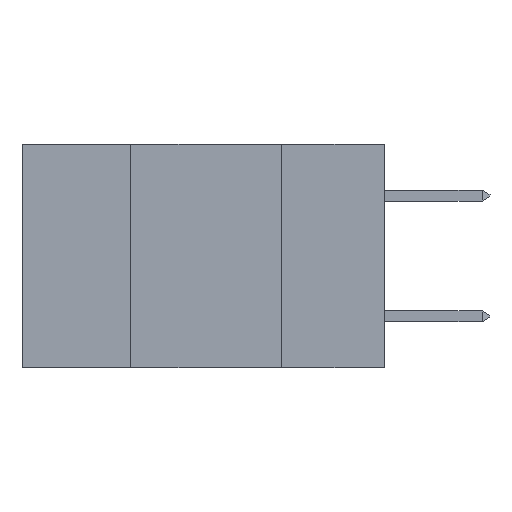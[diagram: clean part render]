
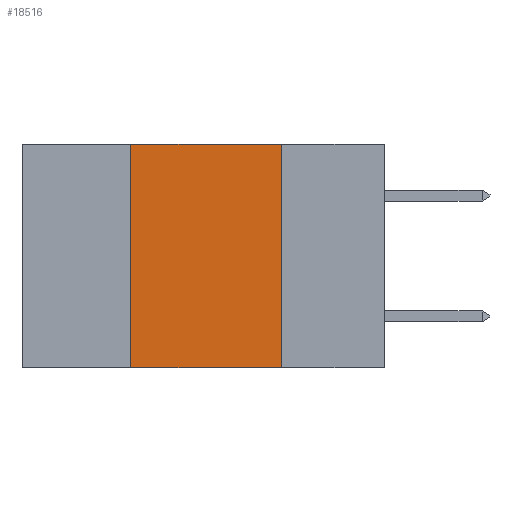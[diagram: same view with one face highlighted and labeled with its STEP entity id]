
A CAD part, left-side view. The second image highlights one B-rep face of the part: STEP entity #18516.
In plain terms, the highlighted planar face has unit normal (-1, 0, 0).
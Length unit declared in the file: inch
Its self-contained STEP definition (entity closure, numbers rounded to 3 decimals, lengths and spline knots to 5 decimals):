
#1096 = LINE ( 'NONE', #18231, #2732 ) ;
#1862 = DIRECTION ( 'NONE',  ( 0., 0., 1. ) ) ;
#2732 = VECTOR ( 'NONE', #21610, 39.37008 ) ;
#2871 = ORIENTED_EDGE ( 'NONE', *, *, #7036, .F. ) ;
#2920 = LINE ( 'NONE', #2976, #15024 ) ;
#2976 = CARTESIAN_POINT ( 'NONE',  ( 0., 0.17, 0. ) ) ;
#3506 = EDGE_CURVE ( 'NONE', #19557, #21065, #7070, .T. ) ;
#3613 = VECTOR ( 'NONE', #1862, 39.37008 ) ;
#3697 = FACE_OUTER_BOUND ( 'NONE', #12694, .T. ) ;
#4032 = DIRECTION ( 'NONE',  ( 0., -1., 0. ) ) ;
#5654 = CARTESIAN_POINT ( 'NONE',  ( 0., 0.6, 0. ) ) ;
#6353 = CARTESIAN_POINT ( 'NONE',  ( 0., 0.6, 0. ) ) ;
#7036 = EDGE_CURVE ( 'NONE', #21065, #18867, #2920, .T. ) ;
#7070 = LINE ( 'NONE', #5654, #15033 ) ;
#7922 = DIRECTION ( 'NONE',  ( 1., 0., 0. ) ) ;
#8069 = DIRECTION ( 'NONE',  ( 0., 0., -1. ) ) ;
#8306 = LINE ( 'NONE', #14078, #3613 ) ;
#8861 = AXIS2_PLACEMENT_3D ( 'NONE', #6353, #7922, #8069 ) ;
#9609 = PLANE ( 'NONE',  #8861 ) ;
#10303 = CARTESIAN_POINT ( 'NONE',  ( 0., 0.17, -0.37 ) ) ;
#10659 = ORIENTED_EDGE ( 'NONE', *, *, #20138, .F. ) ;
#11064 = CARTESIAN_POINT ( 'NONE',  ( 0., 0.17, 0. ) ) ;
#12694 = EDGE_LOOP ( 'NONE', ( #2871, #20544, #10659, #18082 ) ) ;
#14078 = CARTESIAN_POINT ( 'NONE',  ( 0., 0.42, 0. ) ) ;
#15024 = VECTOR ( 'NONE', #15264, 39.37008 ) ;
#15033 = VECTOR ( 'NONE', #4032, 39.37008 ) ;
#15264 = DIRECTION ( 'NONE',  ( 0., 0., -1. ) ) ;
#17601 = VERTEX_POINT ( 'NONE', #18396 ) ;
#18082 = ORIENTED_EDGE ( 'NONE', *, *, #22385, .T. ) ;
#18231 = CARTESIAN_POINT ( 'NONE',  ( 0., 0.6, -0.37 ) ) ;
#18396 = CARTESIAN_POINT ( 'NONE',  ( 0., 0.42, -0.37 ) ) ;
#18516 = ADVANCED_FACE ( 'NONE', ( #3697 ), #9609, .F. ) ;
#18867 = VERTEX_POINT ( 'NONE', #10303 ) ;
#19557 = VERTEX_POINT ( 'NONE', #21289 ) ;
#20138 = EDGE_CURVE ( 'NONE', #17601, #19557, #8306, .T. ) ;
#20544 = ORIENTED_EDGE ( 'NONE', *, *, #3506, .F. ) ;
#21065 = VERTEX_POINT ( 'NONE', #11064 ) ;
#21289 = CARTESIAN_POINT ( 'NONE',  ( 0., 0.42, 0. ) ) ;
#21610 = DIRECTION ( 'NONE',  ( 0., -1., 0. ) ) ;
#22385 = EDGE_CURVE ( 'NONE', #17601, #18867, #1096, .T. ) ;
